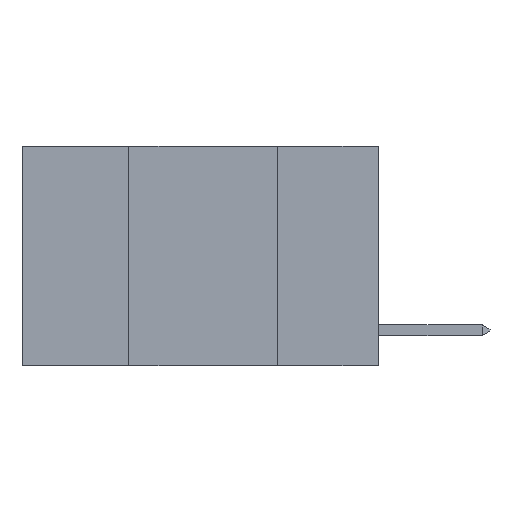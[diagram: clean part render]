
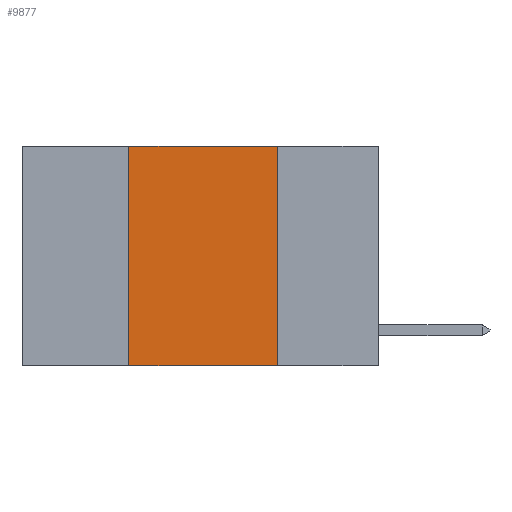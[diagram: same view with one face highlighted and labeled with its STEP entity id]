
A CAD part, left-side view. The second image highlights one B-rep face of the part: STEP entity #9877.
In plain terms, the highlighted planar face has unit normal (-1, 0, 0).
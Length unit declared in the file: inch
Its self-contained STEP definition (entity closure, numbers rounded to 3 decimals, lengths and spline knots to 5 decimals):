
#496 = VERTEX_POINT ( 'NONE', #12537 ) ;
#1057 = EDGE_CURVE ( 'NONE', #15172, #496, #12897, .T. ) ;
#1133 = LINE ( 'NONE', #9234, #15136 ) ;
#1166 = VECTOR ( 'NONE', #5196, 39.37008 ) ;
#4161 = VERTEX_POINT ( 'NONE', #6871 ) ;
#4678 = EDGE_CURVE ( 'NONE', #496, #11916, #16730, .T. ) ;
#4814 = ORIENTED_EDGE ( 'NONE', *, *, #12042, .T. ) ;
#4930 = DIRECTION ( 'NONE',  ( 0., 0., -1. ) ) ;
#4935 = DIRECTION ( 'NONE',  ( 0., -1., 0. ) ) ;
#5196 = DIRECTION ( 'NONE',  ( 0., 0., 1. ) ) ;
#6165 = LINE ( 'NONE', #10518, #1166 ) ;
#6347 = ORIENTED_EDGE ( 'NONE', *, *, #4678, .F. ) ;
#6365 = FACE_OUTER_BOUND ( 'NONE', #7883, .T. ) ;
#6671 = DIRECTION ( 'NONE',  ( 1., 0., 0. ) ) ;
#6861 = CARTESIAN_POINT ( 'NONE',  ( 0., 0.6, 0. ) ) ;
#6871 = CARTESIAN_POINT ( 'NONE',  ( 0., 0.42, -0.37 ) ) ;
#7648 = CARTESIAN_POINT ( 'NONE',  ( 0., 0.17, -0.37 ) ) ;
#7816 = DIRECTION ( 'NONE',  ( 0., -1., 0. ) ) ;
#7883 = EDGE_LOOP ( 'NONE', ( #6347, #10814, #10302, #4814 ) ) ;
#9234 = CARTESIAN_POINT ( 'NONE',  ( 0., 0.6, -0.37 ) ) ;
#9877 = ADVANCED_FACE ( 'NONE', ( #6365 ), #10917, .F. ) ;
#9962 = CARTESIAN_POINT ( 'NONE',  ( 0., 0.42, 0. ) ) ;
#10084 = VECTOR ( 'NONE', #4930, 39.37008 ) ;
#10302 = ORIENTED_EDGE ( 'NONE', *, *, #17117, .F. ) ;
#10518 = CARTESIAN_POINT ( 'NONE',  ( 0., 0.42, 0. ) ) ;
#10814 = ORIENTED_EDGE ( 'NONE', *, *, #1057, .F. ) ;
#10917 = PLANE ( 'NONE',  #13364 ) ;
#11916 = VERTEX_POINT ( 'NONE', #7648 ) ;
#12042 = EDGE_CURVE ( 'NONE', #4161, #11916, #1133, .T. ) ;
#12537 = CARTESIAN_POINT ( 'NONE',  ( 0., 0.17, 0. ) ) ;
#12897 = LINE ( 'NONE', #14642, #13299 ) ;
#12976 = CARTESIAN_POINT ( 'NONE',  ( 0., 0.17, 0. ) ) ;
#13299 = VECTOR ( 'NONE', #7816, 39.37008 ) ;
#13364 = AXIS2_PLACEMENT_3D ( 'NONE', #6861, #6671, #16253 ) ;
#14642 = CARTESIAN_POINT ( 'NONE',  ( 0., 0.6, 0. ) ) ;
#15136 = VECTOR ( 'NONE', #4935, 39.37008 ) ;
#15172 = VERTEX_POINT ( 'NONE', #9962 ) ;
#16253 = DIRECTION ( 'NONE',  ( 0., 0., -1. ) ) ;
#16730 = LINE ( 'NONE', #12976, #10084 ) ;
#17117 = EDGE_CURVE ( 'NONE', #4161, #15172, #6165, .T. ) ;
